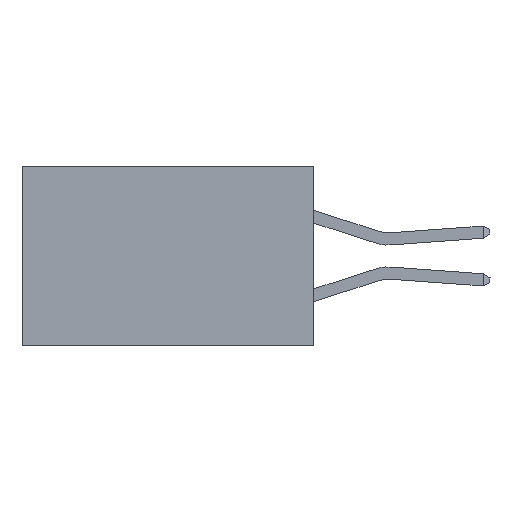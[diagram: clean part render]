
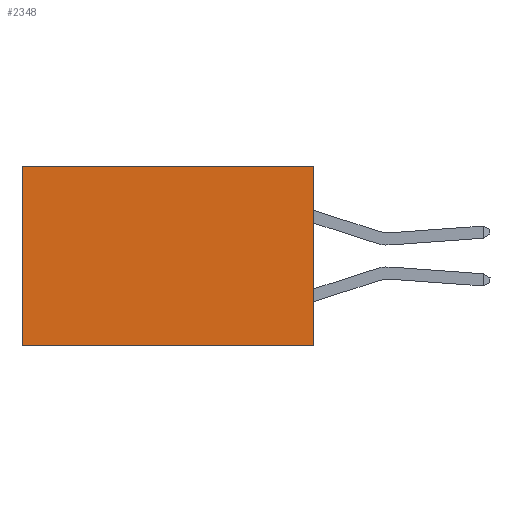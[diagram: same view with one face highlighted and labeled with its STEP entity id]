
A CAD part, left-side view. The second image highlights one B-rep face of the part: STEP entity #2348.
In plain terms, the highlighted planar face has unit normal (-1, 0, 0).
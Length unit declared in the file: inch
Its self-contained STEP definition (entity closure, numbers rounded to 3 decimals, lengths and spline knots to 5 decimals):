
#176 = EDGE_CURVE ( 'NONE', #6031, #1492, #6212, .T. ) ;
#445 = VECTOR ( 'NONE', #6918, 39.37008 ) ;
#529 = EDGE_CURVE ( 'NONE', #8638, #3122, #992, .T. ) ;
#907 = CARTESIAN_POINT ( 'NONE',  ( 0.2875, 0., 0. ) ) ;
#977 = ORIENTED_EDGE ( 'NONE', *, *, #1649, .F. ) ;
#992 = LINE ( 'NONE', #5387, #5664 ) ;
#1123 = ORIENTED_EDGE ( 'NONE', *, *, #529, .F. ) ;
#1257 = DIRECTION ( 'NONE',  ( 1., 0., 0. ) ) ;
#1318 = FACE_OUTER_BOUND ( 'NONE', #6359, .T. ) ;
#1440 = CARTESIAN_POINT ( 'NONE',  ( 0.2875, 0.6, -0.37 ) ) ;
#1492 = VERTEX_POINT ( 'NONE', #1440 ) ;
#1649 = EDGE_CURVE ( 'NONE', #3122, #1492, #8471, .T. ) ;
#1759 = PLANE ( 'NONE',  #6677 ) ;
#2046 = CARTESIAN_POINT ( 'NONE',  ( 0.2875, 0., -0.37 ) ) ;
#2348 = ADVANCED_FACE ( 'NONE', ( #1318 ), #1759, .F. ) ;
#3122 = VERTEX_POINT ( 'NONE', #2046 ) ;
#3727 = VECTOR ( 'NONE', #7580, 39.37008 ) ;
#3744 = CARTESIAN_POINT ( 'NONE',  ( 0.2875, 0.6, 0. ) ) ;
#3960 = CARTESIAN_POINT ( 'NONE',  ( 0.2875, 0., -0.37 ) ) ;
#3994 = DIRECTION ( 'NONE',  ( 0., 0., -1. ) ) ;
#4178 = CARTESIAN_POINT ( 'NONE',  ( 0.2875, 0.6, 0. ) ) ;
#4426 = VECTOR ( 'NONE', #8779, 39.37008 ) ;
#4745 = EDGE_CURVE ( 'NONE', #8638, #6031, #6816, .T. ) ;
#5387 = CARTESIAN_POINT ( 'NONE',  ( 0.2875, 0., 0. ) ) ;
#5664 = VECTOR ( 'NONE', #3994, 39.37008 ) ;
#6031 = VERTEX_POINT ( 'NONE', #4178 ) ;
#6212 = LINE ( 'NONE', #3744, #4426 ) ;
#6359 = EDGE_LOOP ( 'NONE', ( #6634, #977, #1123, #7730 ) ) ;
#6634 = ORIENTED_EDGE ( 'NONE', *, *, #176, .T. ) ;
#6677 = AXIS2_PLACEMENT_3D ( 'NONE', #7576, #1257, #9153 ) ;
#6816 = LINE ( 'NONE', #8350, #445 ) ;
#6918 = DIRECTION ( 'NONE',  ( 0., 1., 0. ) ) ;
#7576 = CARTESIAN_POINT ( 'NONE',  ( 0.2875, 0., 0. ) ) ;
#7580 = DIRECTION ( 'NONE',  ( 0., 1., 0. ) ) ;
#7730 = ORIENTED_EDGE ( 'NONE', *, *, #4745, .T. ) ;
#8350 = CARTESIAN_POINT ( 'NONE',  ( 0.2875, 0., 0. ) ) ;
#8471 = LINE ( 'NONE', #3960, #3727 ) ;
#8638 = VERTEX_POINT ( 'NONE', #907 ) ;
#8779 = DIRECTION ( 'NONE',  ( 0., 0., -1. ) ) ;
#9153 = DIRECTION ( 'NONE',  ( 0., 0., -1. ) ) ;
